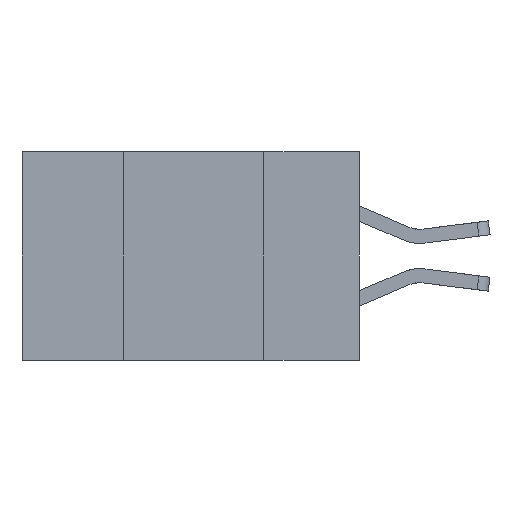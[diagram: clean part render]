
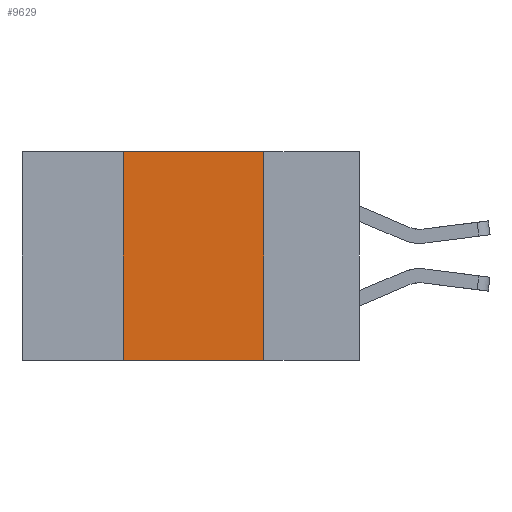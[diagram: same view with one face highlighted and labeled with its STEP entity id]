
A CAD part, left-side view. The second image highlights one B-rep face of the part: STEP entity #9629.
In plain terms, the highlighted planar face has unit normal (-1, 0, 0).
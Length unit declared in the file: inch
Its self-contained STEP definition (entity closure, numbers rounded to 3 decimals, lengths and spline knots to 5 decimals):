
#329 = DIRECTION ( 'NONE',  ( 0., -1., 0. ) ) ;
#1487 = CARTESIAN_POINT ( 'NONE',  ( 0., 0.42, 0. ) ) ;
#1607 = VECTOR ( 'NONE', #329, 39.37008 ) ;
#2264 = ORIENTED_EDGE ( 'NONE', *, *, #9213, .F. ) ;
#2492 = CARTESIAN_POINT ( 'NONE',  ( 0., 0.17, 0. ) ) ;
#2844 = VECTOR ( 'NONE', #14188, 39.37008 ) ;
#3828 = EDGE_CURVE ( 'NONE', #11732, #7982, #13758, .T. ) ;
#4154 = LINE ( 'NONE', #11835, #2844 ) ;
#4203 = DIRECTION ( 'NONE',  ( 0., 0., -1. ) ) ;
#4428 = CARTESIAN_POINT ( 'NONE',  ( 0., 0.17, 0. ) ) ;
#5245 = CARTESIAN_POINT ( 'NONE',  ( 0., 0.42, 0. ) ) ;
#5661 = LINE ( 'NONE', #2492, #11390 ) ;
#5808 = FACE_OUTER_BOUND ( 'NONE', #11726, .T. ) ;
#5936 = CARTESIAN_POINT ( 'NONE',  ( 0., 0.42, -0.37 ) ) ;
#6240 = VERTEX_POINT ( 'NONE', #1487 ) ;
#6248 = DIRECTION ( 'NONE',  ( 0., 0., 1. ) ) ;
#6898 = DIRECTION ( 'NONE',  ( 0., 0., -1. ) ) ;
#6935 = VERTEX_POINT ( 'NONE', #4428 ) ;
#6972 = CARTESIAN_POINT ( 'NONE',  ( 0., 0.17, -0.37 ) ) ;
#7132 = CARTESIAN_POINT ( 'NONE',  ( 0., 0.6, -0.37 ) ) ;
#7252 = CARTESIAN_POINT ( 'NONE',  ( 0., 0.6, 0. ) ) ;
#7982 = VERTEX_POINT ( 'NONE', #6972 ) ;
#8182 = AXIS2_PLACEMENT_3D ( 'NONE', #7252, #8478, #4203 ) ;
#8317 = EDGE_CURVE ( 'NONE', #6935, #7982, #5661, .T. ) ;
#8478 = DIRECTION ( 'NONE',  ( 1., 0., 0. ) ) ;
#9213 = EDGE_CURVE ( 'NONE', #11732, #6240, #12874, .T. ) ;
#9522 = ORIENTED_EDGE ( 'NONE', *, *, #10531, .F. ) ;
#9629 = ADVANCED_FACE ( 'NONE', ( #5808 ), #10736, .F. ) ;
#10531 = EDGE_CURVE ( 'NONE', #6240, #6935, #4154, .T. ) ;
#10736 = PLANE ( 'NONE',  #8182 ) ;
#11260 = ORIENTED_EDGE ( 'NONE', *, *, #3828, .T. ) ;
#11390 = VECTOR ( 'NONE', #6898, 39.37008 ) ;
#11726 = EDGE_LOOP ( 'NONE', ( #11932, #9522, #2264, #11260 ) ) ;
#11732 = VERTEX_POINT ( 'NONE', #5936 ) ;
#11835 = CARTESIAN_POINT ( 'NONE',  ( 0., 0.6, 0. ) ) ;
#11869 = VECTOR ( 'NONE', #6248, 39.37008 ) ;
#11932 = ORIENTED_EDGE ( 'NONE', *, *, #8317, .F. ) ;
#12874 = LINE ( 'NONE', #5245, #11869 ) ;
#13758 = LINE ( 'NONE', #7132, #1607 ) ;
#14188 = DIRECTION ( 'NONE',  ( 0., -1., 0. ) ) ;
